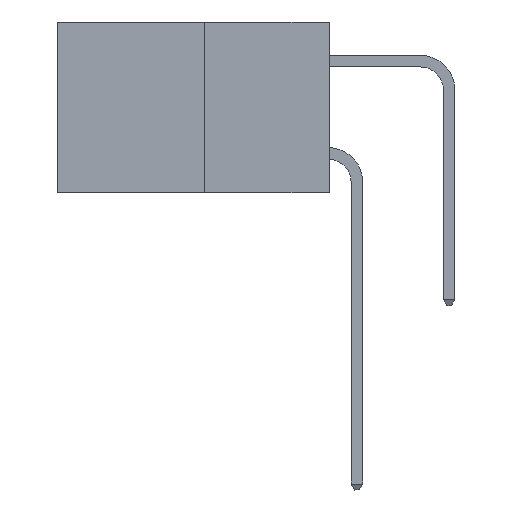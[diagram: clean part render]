
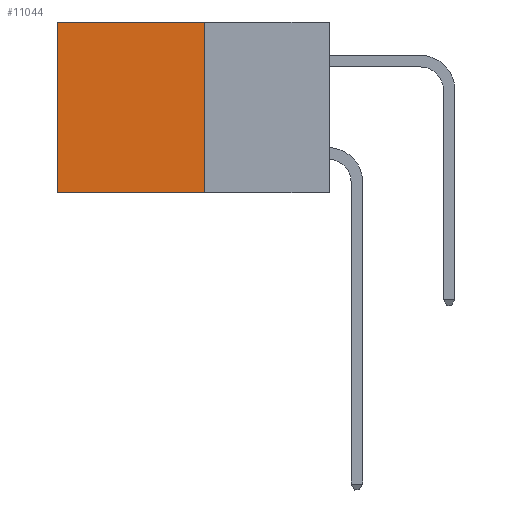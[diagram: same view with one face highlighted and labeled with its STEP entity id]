
A CAD part, left-side view. The second image highlights one B-rep face of the part: STEP entity #11044.
In plain terms, the highlighted planar face has unit normal (-1, 0, 0).
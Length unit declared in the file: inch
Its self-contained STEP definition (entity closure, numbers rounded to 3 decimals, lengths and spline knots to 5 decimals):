
#265 = DIRECTION ( 'NONE',  ( 0., 1., 0. ) ) ;
#329 = PLANE ( 'NONE',  #5895 ) ;
#1504 = VECTOR ( 'NONE', #24201, 39.37008 ) ;
#3633 = LINE ( 'NONE', #7746, #4262 ) ;
#3670 = EDGE_CURVE ( 'NONE', #8361, #8053, #6879, .T. ) ;
#4262 = VECTOR ( 'NONE', #25980, 39.37008 ) ;
#4383 = DIRECTION ( 'NONE',  ( 0., 0., -1. ) ) ;
#5372 = EDGE_CURVE ( 'NONE', #5683, #7478, #14445, .T. ) ;
#5650 = ORIENTED_EDGE ( 'NONE', *, *, #20563, .F. ) ;
#5683 = VERTEX_POINT ( 'NONE', #16691 ) ;
#5895 = AXIS2_PLACEMENT_3D ( 'NONE', #14472, #16540, #4383 ) ;
#6193 = CARTESIAN_POINT ( 'NONE',  ( 0.277, 0.59, 0. ) ) ;
#6879 = LINE ( 'NONE', #25848, #1504 ) ;
#7323 = CARTESIAN_POINT ( 'NONE',  ( 0.277, 0.27, -0.37 ) ) ;
#7478 = VERTEX_POINT ( 'NONE', #7323 ) ;
#7746 = CARTESIAN_POINT ( 'NONE',  ( 0.277, 0.27, 0. ) ) ;
#8053 = VERTEX_POINT ( 'NONE', #25721 ) ;
#8361 = VERTEX_POINT ( 'NONE', #6193 ) ;
#9674 = VECTOR ( 'NONE', #11273, 39.37008 ) ;
#10438 = EDGE_LOOP ( 'NONE', ( #11603, #5650, #17925, #17051 ) ) ;
#10654 = CARTESIAN_POINT ( 'NONE',  ( 0.277, 0.27, -0.37 ) ) ;
#10786 = EDGE_CURVE ( 'NONE', #5683, #8361, #3633, .T. ) ;
#11044 = ADVANCED_FACE ( 'NONE', ( #13428 ), #329, .F. ) ;
#11273 = DIRECTION ( 'NONE',  ( 0., 0., -1. ) ) ;
#11603 = ORIENTED_EDGE ( 'NONE', *, *, #3670, .T. ) ;
#12929 = LINE ( 'NONE', #18560, #24444 ) ;
#13428 = FACE_OUTER_BOUND ( 'NONE', #10438, .T. ) ;
#14445 = LINE ( 'NONE', #10654, #9674 ) ;
#14472 = CARTESIAN_POINT ( 'NONE',  ( 0.277, 0.27, -0.37 ) ) ;
#16540 = DIRECTION ( 'NONE',  ( 1., 0., 0. ) ) ;
#16691 = CARTESIAN_POINT ( 'NONE',  ( 0.277, 0.27, 0. ) ) ;
#17051 = ORIENTED_EDGE ( 'NONE', *, *, #10786, .T. ) ;
#17925 = ORIENTED_EDGE ( 'NONE', *, *, #5372, .F. ) ;
#18560 = CARTESIAN_POINT ( 'NONE',  ( 0.277, 0.27, -0.37 ) ) ;
#20563 = EDGE_CURVE ( 'NONE', #7478, #8053, #12929, .T. ) ;
#24201 = DIRECTION ( 'NONE',  ( 0., 0., -1. ) ) ;
#24444 = VECTOR ( 'NONE', #265, 39.37008 ) ;
#25721 = CARTESIAN_POINT ( 'NONE',  ( 0.277, 0.59, -0.37 ) ) ;
#25848 = CARTESIAN_POINT ( 'NONE',  ( 0.277, 0.59, -0.37 ) ) ;
#25980 = DIRECTION ( 'NONE',  ( 0., 1., 0. ) ) ;
